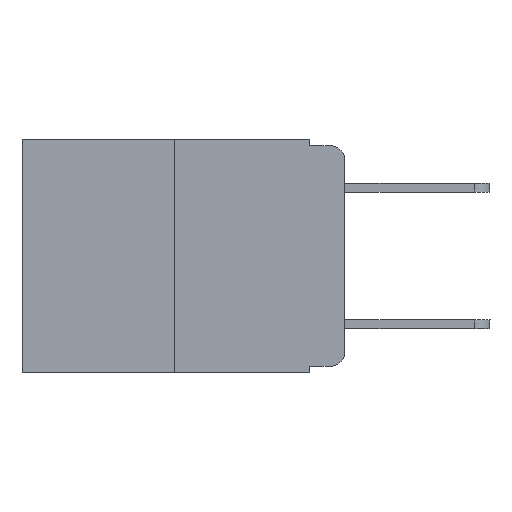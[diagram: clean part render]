
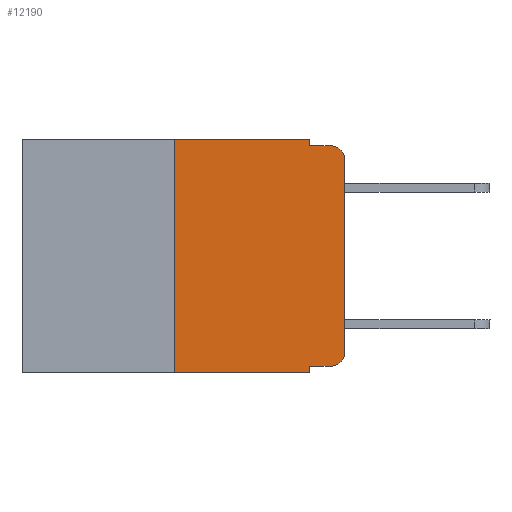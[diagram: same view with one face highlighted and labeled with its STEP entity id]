
A CAD part, left-side view. The second image highlights one B-rep face of the part: STEP entity #12190.
In plain terms, the highlighted planar face has unit normal (-1, 0, 0).
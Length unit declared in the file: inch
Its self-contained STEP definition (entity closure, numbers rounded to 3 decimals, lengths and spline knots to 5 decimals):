
#14 = EDGE_CURVE ( 'NONE', #71, #7897, #8907, .T. ) ;
#71 = VERTEX_POINT ( 'NONE', #5180 ) ;
#127 = CARTESIAN_POINT ( 'NONE',  ( 0., 0.051, -0.01 ) ) ;
#264 = DIRECTION ( 'NONE',  ( 0., 0., -1. ) ) ;
#486 = CARTESIAN_POINT ( 'NONE',  ( 0., 0.473, 0. ) ) ;
#1215 = DIRECTION ( 'NONE',  ( 0., 0., -1. ) ) ;
#1291 = CARTESIAN_POINT ( 'NONE',  ( 0., 0.25, -0.343 ) ) ;
#1312 = DIRECTION ( 'NONE',  ( -1., 0., 0. ) ) ;
#1366 = DIRECTION ( 'NONE',  ( 0., 0., -1. ) ) ;
#1836 = EDGE_CURVE ( 'NONE', #14268, #11791, #19947, .T. ) ;
#2049 = ORIENTED_EDGE ( 'NONE', *, *, #8151, .T. ) ;
#2056 = ORIENTED_EDGE ( 'NONE', *, *, #1836, .F. ) ;
#2169 = DIRECTION ( 'NONE',  ( 0., -1., 0. ) ) ;
#2913 = LINE ( 'NONE', #15605, #6845 ) ;
#3443 = CIRCLE ( 'NONE', #5135, 0.02 ) ;
#3466 = CARTESIAN_POINT ( 'NONE',  ( 0., 0.25, 0. ) ) ;
#3832 = EDGE_CURVE ( 'NONE', #17643, #8247, #14204, .T. ) ;
#3898 = DIRECTION ( 'NONE',  ( 0., 0., 1. ) ) ;
#4470 = LINE ( 'NONE', #20866, #11675 ) ;
#5133 = DIRECTION ( 'NONE',  ( 1., 0., 0. ) ) ;
#5135 = AXIS2_PLACEMENT_3D ( 'NONE', #19182, #1312, #1215 ) ;
#5180 = CARTESIAN_POINT ( 'NONE',  ( 0., 0.051, 0. ) ) ;
#5276 = LINE ( 'NONE', #8319, #19979 ) ;
#5454 = ORIENTED_EDGE ( 'NONE', *, *, #3832, .T. ) ;
#5494 = EDGE_LOOP ( 'NONE', ( #5454, #10011, #14274, #6441, #10514, #2056, #2049, #14951, #19862, #10476 ) ) ;
#5559 = LINE ( 'NONE', #486, #19270 ) ;
#5571 = CARTESIAN_POINT ( 'NONE',  ( 0., 0.25, 0. ) ) ;
#5983 = CARTESIAN_POINT ( 'NONE',  ( 0., 0.02, -0.03 ) ) ;
#6018 = CARTESIAN_POINT ( 'NONE',  ( 0., 0.051, -0.01 ) ) ;
#6175 = VERTEX_POINT ( 'NONE', #6256 ) ;
#6256 = CARTESIAN_POINT ( 'NONE',  ( 0., 0.02, -0.01 ) ) ;
#6422 = VECTOR ( 'NONE', #6559, 39.37008 ) ;
#6441 = ORIENTED_EDGE ( 'NONE', *, *, #14, .F. ) ;
#6559 = DIRECTION ( 'NONE',  ( 0., -1., 0. ) ) ;
#6845 = VECTOR ( 'NONE', #10625, 39.37008 ) ;
#7470 = EDGE_CURVE ( 'NONE', #9266, #14225, #4470, .T. ) ;
#7735 = CARTESIAN_POINT ( 'NONE',  ( 0., 0.051, -0.333 ) ) ;
#7897 = VERTEX_POINT ( 'NONE', #6018 ) ;
#8101 = AXIS2_PLACEMENT_3D ( 'NONE', #5983, #14121, #17516 ) ;
#8126 = VERTEX_POINT ( 'NONE', #10117 ) ;
#8151 = EDGE_CURVE ( 'NONE', #14268, #8126, #5276, .T. ) ;
#8247 = VERTEX_POINT ( 'NONE', #20165 ) ;
#8319 = CARTESIAN_POINT ( 'NONE',  ( 0., 0.473, -0.343 ) ) ;
#8907 = LINE ( 'NONE', #20623, #18460 ) ;
#9266 = VERTEX_POINT ( 'NONE', #7735 ) ;
#9873 = FACE_OUTER_BOUND ( 'NONE', #5494, .T. ) ;
#10011 = ORIENTED_EDGE ( 'NONE', *, *, #15213, .T. ) ;
#10117 = CARTESIAN_POINT ( 'NONE',  ( 0., 0.051, -0.343 ) ) ;
#10198 = CARTESIAN_POINT ( 'NONE',  ( 0., 0.02, -0.333 ) ) ;
#10476 = ORIENTED_EDGE ( 'NONE', *, *, #11987, .T. ) ;
#10514 = ORIENTED_EDGE ( 'NONE', *, *, #15453, .F. ) ;
#10625 = DIRECTION ( 'NONE',  ( 0., 0., -1. ) ) ;
#11019 = CARTESIAN_POINT ( 'NONE',  ( 0., 0., 0. ) ) ;
#11675 = VECTOR ( 'NONE', #16099, 39.37008 ) ;
#11791 = VERTEX_POINT ( 'NONE', #5571 ) ;
#11987 = EDGE_CURVE ( 'NONE', #14225, #17643, #3443, .T. ) ;
#12190 = ADVANCED_FACE ( 'NONE', ( #9873 ), #14743, .F. ) ;
#14121 = DIRECTION ( 'NONE',  ( -1., 0., 0. ) ) ;
#14204 = LINE ( 'NONE', #11019, #19595 ) ;
#14225 = VERTEX_POINT ( 'NONE', #10198 ) ;
#14268 = VERTEX_POINT ( 'NONE', #1291 ) ;
#14274 = ORIENTED_EDGE ( 'NONE', *, *, #15001, .F. ) ;
#14743 = PLANE ( 'NONE',  #17609 ) ;
#14780 = DIRECTION ( 'NONE',  ( 0., -1., 0. ) ) ;
#14951 = ORIENTED_EDGE ( 'NONE', *, *, #19575, .F. ) ;
#15001 = EDGE_CURVE ( 'NONE', #7897, #6175, #17780, .T. ) ;
#15213 = EDGE_CURVE ( 'NONE', #8247, #6175, #15220, .T. ) ;
#15220 = CIRCLE ( 'NONE', #8101, 0.02 ) ;
#15453 = EDGE_CURVE ( 'NONE', #11791, #71, #5559, .T. ) ;
#15605 = CARTESIAN_POINT ( 'NONE',  ( 0., 0.051, 0. ) ) ;
#16099 = DIRECTION ( 'NONE',  ( 0., -1., 0. ) ) ;
#17232 = VECTOR ( 'NONE', #3898, 39.37008 ) ;
#17489 = DIRECTION ( 'NONE',  ( 0., 0., 1. ) ) ;
#17516 = DIRECTION ( 'NONE',  ( 0., 0., -1. ) ) ;
#17609 = AXIS2_PLACEMENT_3D ( 'NONE', #18518, #5133, #264 ) ;
#17643 = VERTEX_POINT ( 'NONE', #17659 ) ;
#17659 = CARTESIAN_POINT ( 'NONE',  ( 0., 0., -0.313 ) ) ;
#17780 = LINE ( 'NONE', #127, #6422 ) ;
#18460 = VECTOR ( 'NONE', #1366, 39.37008 ) ;
#18518 = CARTESIAN_POINT ( 'NONE',  ( 0., 0.473, 0. ) ) ;
#19182 = CARTESIAN_POINT ( 'NONE',  ( 0., 0.02, -0.313 ) ) ;
#19270 = VECTOR ( 'NONE', #2169, 39.37008 ) ;
#19575 = EDGE_CURVE ( 'NONE', #9266, #8126, #2913, .T. ) ;
#19595 = VECTOR ( 'NONE', #17489, 39.37008 ) ;
#19862 = ORIENTED_EDGE ( 'NONE', *, *, #7470, .T. ) ;
#19947 = LINE ( 'NONE', #3466, #17232 ) ;
#19979 = VECTOR ( 'NONE', #14780, 39.37008 ) ;
#20165 = CARTESIAN_POINT ( 'NONE',  ( 0., 0., -0.03 ) ) ;
#20623 = CARTESIAN_POINT ( 'NONE',  ( 0., 0.051, 0. ) ) ;
#20866 = CARTESIAN_POINT ( 'NONE',  ( 0., 0.051, -0.333 ) ) ;
